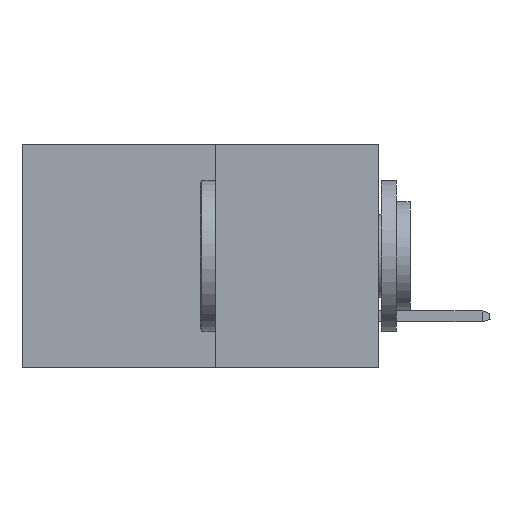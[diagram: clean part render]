
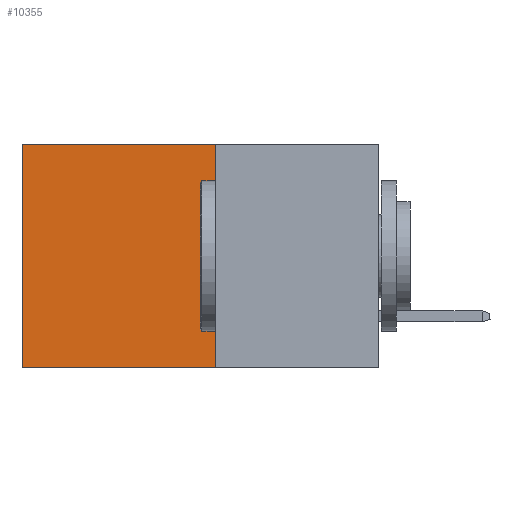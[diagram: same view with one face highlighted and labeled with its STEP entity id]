
A CAD part, left-side view. The second image highlights one B-rep face of the part: STEP entity #10355.
In plain terms, the highlighted planar face has unit normal (-1, 0, 0).
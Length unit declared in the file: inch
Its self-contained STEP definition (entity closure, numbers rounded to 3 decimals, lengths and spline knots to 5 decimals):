
#387 = VERTEX_POINT ( 'NONE', #9545 ) ;
#1034 = DIRECTION ( 'NONE',  ( 0., 1., 0. ) ) ;
#1082 = CARTESIAN_POINT ( 'NONE',  ( 0.277, 0.27, 0. ) ) ;
#1084 = VECTOR ( 'NONE', #1034, 39.37008 ) ;
#1116 = CARTESIAN_POINT ( 'NONE',  ( 0.277, 0.27, 0. ) ) ;
#1128 = DIRECTION ( 'NONE',  ( 0., 0., -1. ) ) ;
#1405 = LINE ( 'NONE', #1116, #1084 ) ;
#1773 = CARTESIAN_POINT ( 'NONE',  ( 0.277, 0.59, -0.37 ) ) ;
#1816 = VECTOR ( 'NONE', #3902, 39.37008 ) ;
#1962 = ORIENTED_EDGE ( 'NONE', *, *, #4344, .T. ) ;
#2122 = CARTESIAN_POINT ( 'NONE',  ( 0.277, 0.27, -0.37 ) ) ;
#2294 = LINE ( 'NONE', #11623, #7283 ) ;
#2730 = EDGE_CURVE ( 'NONE', #4416, #7456, #7741, .T. ) ;
#3259 = VERTEX_POINT ( 'NONE', #6269 ) ;
#3523 = DIRECTION ( 'NONE',  ( 0., 0., -1. ) ) ;
#3902 = DIRECTION ( 'NONE',  ( 0., 0., -1. ) ) ;
#4344 = EDGE_CURVE ( 'NONE', #3259, #387, #5106, .T. ) ;
#4416 = VERTEX_POINT ( 'NONE', #1082 ) ;
#4432 = ORIENTED_EDGE ( 'NONE', *, *, #9355, .F. ) ;
#4788 = ORIENTED_EDGE ( 'NONE', *, *, #2730, .F. ) ;
#5106 = LINE ( 'NONE', #1773, #9706 ) ;
#6269 = CARTESIAN_POINT ( 'NONE',  ( 0.277, 0.59, 0. ) ) ;
#6310 = EDGE_CURVE ( 'NONE', #4416, #3259, #1405, .T. ) ;
#7146 = DIRECTION ( 'NONE',  ( 1., 0., 0. ) ) ;
#7283 = VECTOR ( 'NONE', #12571, 39.37008 ) ;
#7456 = VERTEX_POINT ( 'NONE', #9696 ) ;
#7741 = LINE ( 'NONE', #12438, #1816 ) ;
#9052 = ORIENTED_EDGE ( 'NONE', *, *, #6310, .T. ) ;
#9355 = EDGE_CURVE ( 'NONE', #7456, #387, #2294, .T. ) ;
#9545 = CARTESIAN_POINT ( 'NONE',  ( 0.277, 0.59, -0.37 ) ) ;
#9696 = CARTESIAN_POINT ( 'NONE',  ( 0.277, 0.27, -0.37 ) ) ;
#9706 = VECTOR ( 'NONE', #3523, 39.37008 ) ;
#10355 = ADVANCED_FACE ( 'NONE', ( #10574 ), #10985, .F. ) ;
#10574 = FACE_OUTER_BOUND ( 'NONE', #11883, .T. ) ;
#10985 = PLANE ( 'NONE',  #11477 ) ;
#11477 = AXIS2_PLACEMENT_3D ( 'NONE', #2122, #7146, #1128 ) ;
#11623 = CARTESIAN_POINT ( 'NONE',  ( 0.277, 0.27, -0.37 ) ) ;
#11883 = EDGE_LOOP ( 'NONE', ( #1962, #4432, #4788, #9052 ) ) ;
#12438 = CARTESIAN_POINT ( 'NONE',  ( 0.277, 0.27, -0.37 ) ) ;
#12571 = DIRECTION ( 'NONE',  ( 0., 1., 0. ) ) ;
